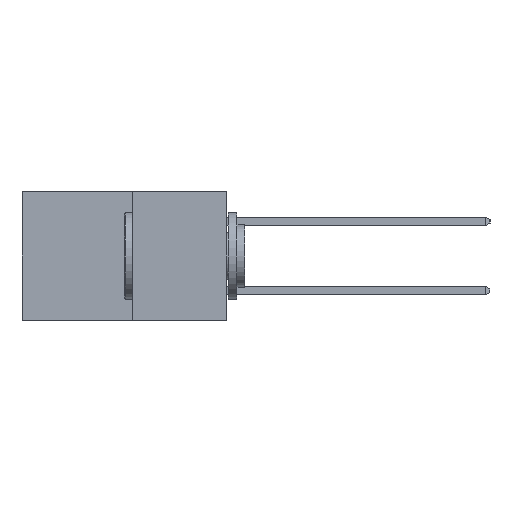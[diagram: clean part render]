
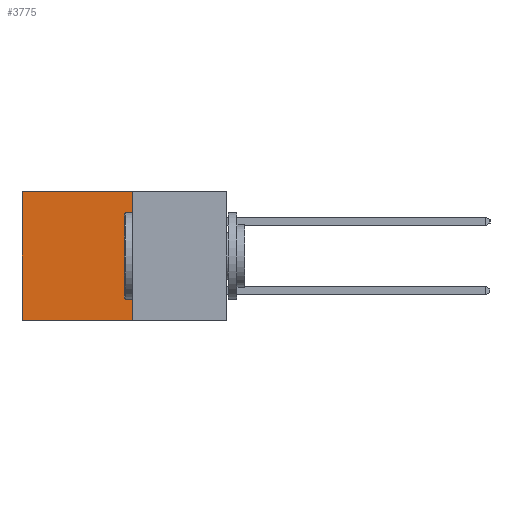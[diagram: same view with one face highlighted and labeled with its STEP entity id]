
A CAD part, left-side view. The second image highlights one B-rep face of the part: STEP entity #3775.
In plain terms, the highlighted planar face has unit normal (-1, 0, 0).
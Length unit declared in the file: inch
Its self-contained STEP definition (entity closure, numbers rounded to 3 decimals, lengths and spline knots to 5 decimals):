
#49 = DIRECTION ( 'NONE',  ( 1., 0., 0. ) ) ;
#323 = CARTESIAN_POINT ( 'NONE',  ( 0.277, 0.27, 0. ) ) ;
#712 = LINE ( 'NONE', #6988, #6399 ) ;
#879 = AXIS2_PLACEMENT_3D ( 'NONE', #4520, #49, #12692 ) ;
#963 = CARTESIAN_POINT ( 'NONE',  ( 0.277, 0.27, -0.37 ) ) ;
#1914 = VERTEX_POINT ( 'NONE', #963 ) ;
#2420 = CARTESIAN_POINT ( 'NONE',  ( 0.277, 0.59, -0.37 ) ) ;
#2525 = VERTEX_POINT ( 'NONE', #2420 ) ;
#3473 = VECTOR ( 'NONE', #5276, 39.37008 ) ;
#3753 = CARTESIAN_POINT ( 'NONE',  ( 0.277, 0.27, -0.37 ) ) ;
#3775 = ADVANCED_FACE ( 'NONE', ( #6767 ), #12662, .F. ) ;
#3932 = DIRECTION ( 'NONE',  ( 0., 0., -1. ) ) ;
#4096 = EDGE_CURVE ( 'NONE', #4449, #1914, #5156, .T. ) ;
#4307 = DIRECTION ( 'NONE',  ( 0., 1., 0. ) ) ;
#4449 = VERTEX_POINT ( 'NONE', #323 ) ;
#4520 = CARTESIAN_POINT ( 'NONE',  ( 0.277, 0.27, -0.37 ) ) ;
#5025 = ORIENTED_EDGE ( 'NONE', *, *, #12814, .T. ) ;
#5131 = CARTESIAN_POINT ( 'NONE',  ( 0.277, 0.27, -0.37 ) ) ;
#5156 = LINE ( 'NONE', #3753, #13934 ) ;
#5276 = DIRECTION ( 'NONE',  ( 0., 1., 0. ) ) ;
#5738 = ORIENTED_EDGE ( 'NONE', *, *, #4096, .F. ) ;
#6167 = LINE ( 'NONE', #12305, #10669 ) ;
#6255 = EDGE_CURVE ( 'NONE', #1914, #2525, #7207, .T. ) ;
#6399 = VECTOR ( 'NONE', #8131, 39.37008 ) ;
#6767 = FACE_OUTER_BOUND ( 'NONE', #8467, .T. ) ;
#6988 = CARTESIAN_POINT ( 'NONE',  ( 0.277, 0.59, -0.37 ) ) ;
#7207 = LINE ( 'NONE', #5131, #3473 ) ;
#8131 = DIRECTION ( 'NONE',  ( 0., 0., -1. ) ) ;
#8467 = EDGE_LOOP ( 'NONE', ( #14354, #10764, #5738, #5025 ) ) ;
#10383 = EDGE_CURVE ( 'NONE', #11890, #2525, #712, .T. ) ;
#10642 = CARTESIAN_POINT ( 'NONE',  ( 0.277, 0.59, 0. ) ) ;
#10669 = VECTOR ( 'NONE', #4307, 39.37008 ) ;
#10764 = ORIENTED_EDGE ( 'NONE', *, *, #6255, .F. ) ;
#11890 = VERTEX_POINT ( 'NONE', #10642 ) ;
#12305 = CARTESIAN_POINT ( 'NONE',  ( 0.277, 0.27, 0. ) ) ;
#12662 = PLANE ( 'NONE',  #879 ) ;
#12692 = DIRECTION ( 'NONE',  ( 0., 0., -1. ) ) ;
#12814 = EDGE_CURVE ( 'NONE', #4449, #11890, #6167, .T. ) ;
#13934 = VECTOR ( 'NONE', #3932, 39.37008 ) ;
#14354 = ORIENTED_EDGE ( 'NONE', *, *, #10383, .T. ) ;
